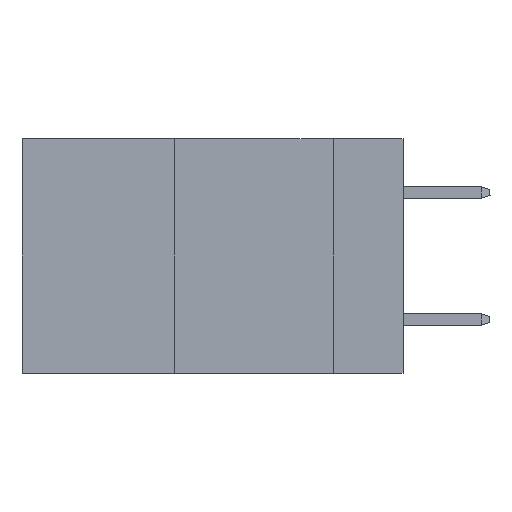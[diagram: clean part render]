
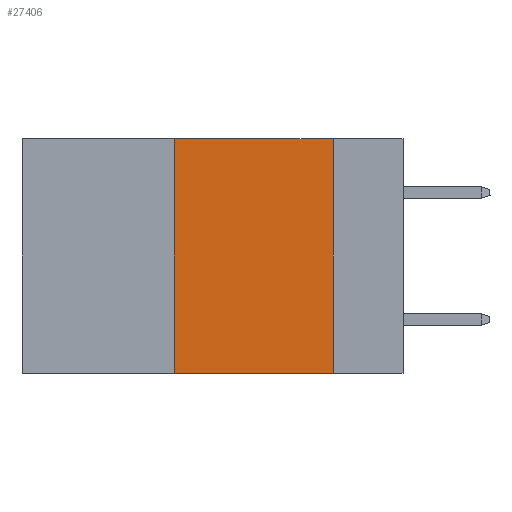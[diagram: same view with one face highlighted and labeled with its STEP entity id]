
A CAD part, left-side view. The second image highlights one B-rep face of the part: STEP entity #27406.
In plain terms, the highlighted planar face has unit normal (-1, 0, 0).
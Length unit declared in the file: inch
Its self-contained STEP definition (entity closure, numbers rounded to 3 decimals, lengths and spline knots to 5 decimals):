
#90 = EDGE_CURVE ( 'NONE', #14922, #21951, #25829, .T. ) ;
#177 = DIRECTION ( 'NONE',  ( 0., 0., 1. ) ) ;
#3386 = EDGE_CURVE ( 'NONE', #15085, #16227, #30092, .T. ) ;
#3597 = CARTESIAN_POINT ( 'NONE',  ( 0., 0.36, -0.37 ) ) ;
#4311 = DIRECTION ( 'NONE',  ( 0., 0., -1. ) ) ;
#5391 = CARTESIAN_POINT ( 'NONE',  ( 0., 0.36, 0. ) ) ;
#5758 = VECTOR ( 'NONE', #4311, 39.37008 ) ;
#5877 = LINE ( 'NONE', #29058, #26317 ) ;
#6184 = CARTESIAN_POINT ( 'NONE',  ( 0., 0.36, 0. ) ) ;
#7701 = ORIENTED_EDGE ( 'NONE', *, *, #24849, .F. ) ;
#8192 = VECTOR ( 'NONE', #36395, 39.37008 ) ;
#9986 = EDGE_CURVE ( 'NONE', #14922, #16227, #19203, .T. ) ;
#12581 = DIRECTION ( 'NONE',  ( 1., 0., 0. ) ) ;
#12735 = CARTESIAN_POINT ( 'NONE',  ( 0., 0.11, 0. ) ) ;
#12775 = PLANE ( 'NONE',  #26975 ) ;
#14066 = CARTESIAN_POINT ( 'NONE',  ( 0., 0.11, -0.37 ) ) ;
#14922 = VERTEX_POINT ( 'NONE', #3597 ) ;
#15085 = VERTEX_POINT ( 'NONE', #12735 ) ;
#15217 = CARTESIAN_POINT ( 'NONE',  ( 0., 0.6, 0. ) ) ;
#15887 = CARTESIAN_POINT ( 'NONE',  ( 0., 0.11, 0. ) ) ;
#16227 = VERTEX_POINT ( 'NONE', #14066 ) ;
#17838 = FACE_OUTER_BOUND ( 'NONE', #26832, .T. ) ;
#19203 = LINE ( 'NONE', #30610, #8192 ) ;
#20025 = ORIENTED_EDGE ( 'NONE', *, *, #9986, .T. ) ;
#20797 = DIRECTION ( 'NONE',  ( 0., -1., 0. ) ) ;
#21951 = VERTEX_POINT ( 'NONE', #5391 ) ;
#24849 = EDGE_CURVE ( 'NONE', #21951, #15085, #5877, .T. ) ;
#24996 = VECTOR ( 'NONE', #177, 39.37008 ) ;
#25829 = LINE ( 'NONE', #6184, #24996 ) ;
#26317 = VECTOR ( 'NONE', #20797, 39.37008 ) ;
#26832 = EDGE_LOOP ( 'NONE', ( #27895, #7701, #29311, #20025 ) ) ;
#26975 = AXIS2_PLACEMENT_3D ( 'NONE', #15217, #12581, #35410 ) ;
#27406 = ADVANCED_FACE ( 'NONE', ( #17838 ), #12775, .F. ) ;
#27895 = ORIENTED_EDGE ( 'NONE', *, *, #3386, .F. ) ;
#29058 = CARTESIAN_POINT ( 'NONE',  ( 0., 0.6, 0. ) ) ;
#29311 = ORIENTED_EDGE ( 'NONE', *, *, #90, .F. ) ;
#30092 = LINE ( 'NONE', #15887, #5758 ) ;
#30610 = CARTESIAN_POINT ( 'NONE',  ( 0., 0.6, -0.37 ) ) ;
#35410 = DIRECTION ( 'NONE',  ( 0., 0., -1. ) ) ;
#36395 = DIRECTION ( 'NONE',  ( 0., -1., 0. ) ) ;
